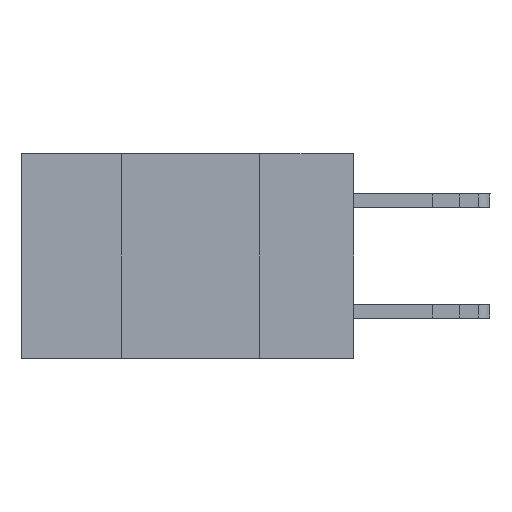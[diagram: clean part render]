
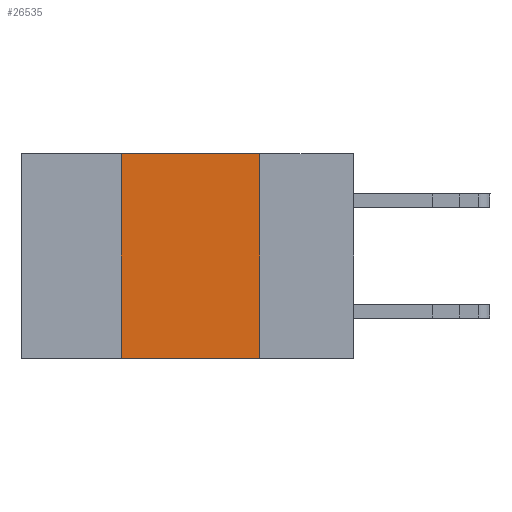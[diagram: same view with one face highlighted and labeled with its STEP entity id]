
A CAD part, left-side view. The second image highlights one B-rep face of the part: STEP entity #26535.
In plain terms, the highlighted planar face has unit normal (-1, 0, 0).
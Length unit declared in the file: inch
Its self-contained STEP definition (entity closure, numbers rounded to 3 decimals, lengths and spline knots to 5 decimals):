
#587 = LINE ( 'NONE', #3119, #30108 ) ;
#624 = ORIENTED_EDGE ( 'NONE', *, *, #3614, .F. ) ;
#2967 = CARTESIAN_POINT ( 'NONE',  ( 0., 0.17, -0.37 ) ) ;
#3119 = CARTESIAN_POINT ( 'NONE',  ( 0., 0.17, 0. ) ) ;
#3255 = CARTESIAN_POINT ( 'NONE',  ( 0., 0.42, 0. ) ) ;
#3614 = EDGE_CURVE ( 'NONE', #17246, #23064, #587, .T. ) ;
#6232 = CARTESIAN_POINT ( 'NONE',  ( 0., 0.6, 0. ) ) ;
#7184 = AXIS2_PLACEMENT_3D ( 'NONE', #6232, #22011, #26932 ) ;
#7410 = DIRECTION ( 'NONE',  ( 0., -1., 0. ) ) ;
#7697 = EDGE_CURVE ( 'NONE', #15297, #13822, #21243, .T. ) ;
#8451 = CARTESIAN_POINT ( 'NONE',  ( 0., 0.17, 0. ) ) ;
#10546 = VECTOR ( 'NONE', #13606, 39.37008 ) ;
#11214 = CARTESIAN_POINT ( 'NONE',  ( 0., 0.42, 0. ) ) ;
#11758 = EDGE_CURVE ( 'NONE', #15297, #23064, #17697, .T. ) ;
#12661 = LINE ( 'NONE', #15358, #25636 ) ;
#13391 = ORIENTED_EDGE ( 'NONE', *, *, #17508, .F. ) ;
#13606 = DIRECTION ( 'NONE',  ( 0., 0., 1. ) ) ;
#13822 = VERTEX_POINT ( 'NONE', #11214 ) ;
#14474 = ORIENTED_EDGE ( 'NONE', *, *, #7697, .F. ) ;
#15087 = CARTESIAN_POINT ( 'NONE',  ( 0., 0.42, -0.37 ) ) ;
#15297 = VERTEX_POINT ( 'NONE', #15087 ) ;
#15358 = CARTESIAN_POINT ( 'NONE',  ( 0., 0.6, 0. ) ) ;
#16673 = DIRECTION ( 'NONE',  ( 0., 0., -1. ) ) ;
#16745 = FACE_OUTER_BOUND ( 'NONE', #29290, .T. ) ;
#17246 = VERTEX_POINT ( 'NONE', #8451 ) ;
#17508 = EDGE_CURVE ( 'NONE', #13822, #17246, #12661, .T. ) ;
#17697 = LINE ( 'NONE', #17868, #31855 ) ;
#17868 = CARTESIAN_POINT ( 'NONE',  ( 0., 0.6, -0.37 ) ) ;
#18650 = ORIENTED_EDGE ( 'NONE', *, *, #11758, .T. ) ;
#21243 = LINE ( 'NONE', #3255, #10546 ) ;
#22011 = DIRECTION ( 'NONE',  ( 1., 0., 0. ) ) ;
#23064 = VERTEX_POINT ( 'NONE', #2967 ) ;
#25636 = VECTOR ( 'NONE', #7410, 39.37008 ) ;
#26535 = ADVANCED_FACE ( 'NONE', ( #16745 ), #29460, .F. ) ;
#26932 = DIRECTION ( 'NONE',  ( 0., 0., -1. ) ) ;
#28037 = DIRECTION ( 'NONE',  ( 0., -1., 0. ) ) ;
#29290 = EDGE_LOOP ( 'NONE', ( #624, #13391, #14474, #18650 ) ) ;
#29460 = PLANE ( 'NONE',  #7184 ) ;
#30108 = VECTOR ( 'NONE', #16673, 39.37008 ) ;
#31855 = VECTOR ( 'NONE', #28037, 39.37008 ) ;
